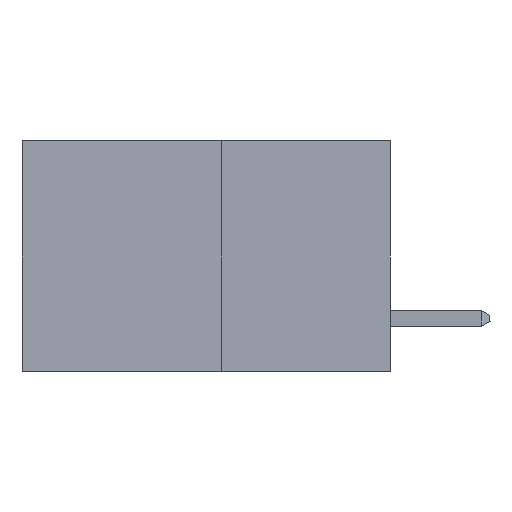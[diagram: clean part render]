
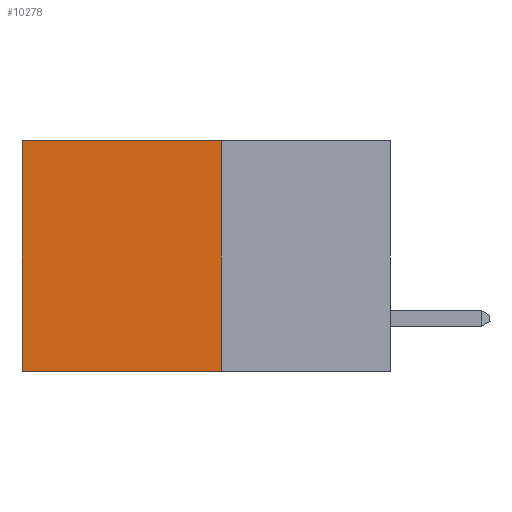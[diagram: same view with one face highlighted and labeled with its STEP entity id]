
A CAD part, left-side view. The second image highlights one B-rep face of the part: STEP entity #10278.
In plain terms, the highlighted planar face has unit normal (-1, 0, 0).
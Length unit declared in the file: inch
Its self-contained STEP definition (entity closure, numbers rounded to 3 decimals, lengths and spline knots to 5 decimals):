
#1410 = CARTESIAN_POINT ( 'NONE',  ( 0.277, 0.27, -0.37 ) ) ;
#1507 = CARTESIAN_POINT ( 'NONE',  ( 0.277, 0.27, -0.37 ) ) ;
#1778 = DIRECTION ( 'NONE',  ( 0., 1., 0. ) ) ;
#2110 = EDGE_CURVE ( 'NONE', #9601, #13365, #6497, .T. ) ;
#2566 = DIRECTION ( 'NONE',  ( 0., 0., -1. ) ) ;
#3415 = EDGE_CURVE ( 'NONE', #5940, #13365, #4727, .T. ) ;
#3517 = VECTOR ( 'NONE', #6431, 39.37008 ) ;
#4422 = EDGE_CURVE ( 'NONE', #8893, #9601, #11143, .T. ) ;
#4512 = EDGE_CURVE ( 'NONE', #8893, #5940, #12703, .T. ) ;
#4584 = ORIENTED_EDGE ( 'NONE', *, *, #3415, .F. ) ;
#4727 = LINE ( 'NONE', #1507, #10661 ) ;
#5195 = VECTOR ( 'NONE', #5930, 39.37008 ) ;
#5420 = CARTESIAN_POINT ( 'NONE',  ( 0.277, 0.27, 0. ) ) ;
#5785 = CARTESIAN_POINT ( 'NONE',  ( 0.277, 0.59, -0.37 ) ) ;
#5881 = CARTESIAN_POINT ( 'NONE',  ( 0.277, 0.27, 0. ) ) ;
#5889 = CARTESIAN_POINT ( 'NONE',  ( 0.277, 0.59, 0. ) ) ;
#5930 = DIRECTION ( 'NONE',  ( 0., 1., 0. ) ) ;
#5940 = VERTEX_POINT ( 'NONE', #10506 ) ;
#6310 = EDGE_LOOP ( 'NONE', ( #12094, #4584, #13470, #10868 ) ) ;
#6431 = DIRECTION ( 'NONE',  ( 0., 0., -1. ) ) ;
#6497 = LINE ( 'NONE', #10603, #3517 ) ;
#6782 = VECTOR ( 'NONE', #8853, 39.37008 ) ;
#8853 = DIRECTION ( 'NONE',  ( 0., 0., -1. ) ) ;
#8893 = VERTEX_POINT ( 'NONE', #5420 ) ;
#8921 = CARTESIAN_POINT ( 'NONE',  ( 0.277, 0.27, -0.37 ) ) ;
#9286 = DIRECTION ( 'NONE',  ( 1., 0., 0. ) ) ;
#9601 = VERTEX_POINT ( 'NONE', #5889 ) ;
#10278 = ADVANCED_FACE ( 'NONE', ( #11696 ), #11495, .F. ) ;
#10506 = CARTESIAN_POINT ( 'NONE',  ( 0.277, 0.27, -0.37 ) ) ;
#10603 = CARTESIAN_POINT ( 'NONE',  ( 0.277, 0.59, -0.37 ) ) ;
#10661 = VECTOR ( 'NONE', #1778, 39.37008 ) ;
#10868 = ORIENTED_EDGE ( 'NONE', *, *, #4422, .T. ) ;
#10977 = AXIS2_PLACEMENT_3D ( 'NONE', #1410, #9286, #2566 ) ;
#11143 = LINE ( 'NONE', #5881, #5195 ) ;
#11495 = PLANE ( 'NONE',  #10977 ) ;
#11696 = FACE_OUTER_BOUND ( 'NONE', #6310, .T. ) ;
#12094 = ORIENTED_EDGE ( 'NONE', *, *, #2110, .T. ) ;
#12703 = LINE ( 'NONE', #8921, #6782 ) ;
#13365 = VERTEX_POINT ( 'NONE', #5785 ) ;
#13470 = ORIENTED_EDGE ( 'NONE', *, *, #4512, .F. ) ;
